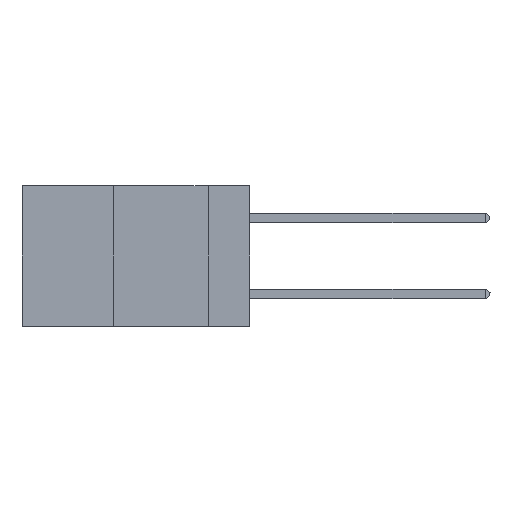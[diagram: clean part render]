
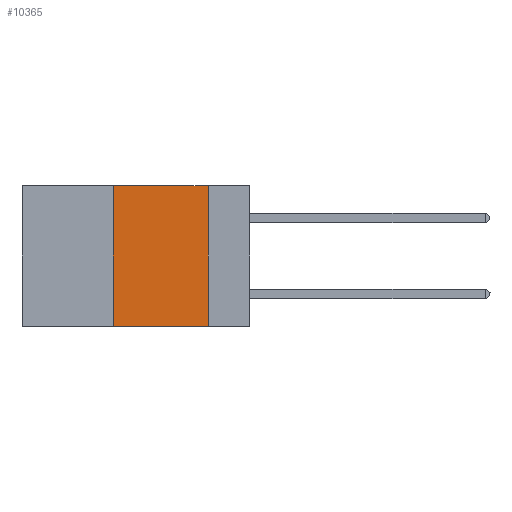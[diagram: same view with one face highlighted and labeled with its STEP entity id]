
A CAD part, left-side view. The second image highlights one B-rep face of the part: STEP entity #10365.
In plain terms, the highlighted planar face has unit normal (-1, 0, 0).
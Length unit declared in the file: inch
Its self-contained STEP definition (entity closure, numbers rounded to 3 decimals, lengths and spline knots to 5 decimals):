
#859 = ORIENTED_EDGE ( 'NONE', *, *, #12280, .F. ) ;
#2120 = CARTESIAN_POINT ( 'NONE',  ( 0., 0.36, 0. ) ) ;
#2125 = DIRECTION ( 'NONE',  ( 0., -1., 0. ) ) ;
#3086 = EDGE_CURVE ( 'NONE', #7713, #8307, #15124, .T. ) ;
#3375 = CARTESIAN_POINT ( 'NONE',  ( 0., 0.36, -0.37 ) ) ;
#3835 = ORIENTED_EDGE ( 'NONE', *, *, #3086, .F. ) ;
#4022 = LINE ( 'NONE', #10146, #11117 ) ;
#5123 = VERTEX_POINT ( 'NONE', #9319 ) ;
#5282 = EDGE_CURVE ( 'NONE', #7713, #5123, #4022, .T. ) ;
#5832 = VECTOR ( 'NONE', #16534, 39.37008 ) ;
#6125 = DIRECTION ( 'NONE',  ( 0., 0., -1. ) ) ;
#6964 = ORIENTED_EDGE ( 'NONE', *, *, #5282, .T. ) ;
#7713 = VERTEX_POINT ( 'NONE', #3375 ) ;
#7771 = EDGE_LOOP ( 'NONE', ( #859, #21436, #3835, #6964 ) ) ;
#8307 = VERTEX_POINT ( 'NONE', #10862 ) ;
#9319 = CARTESIAN_POINT ( 'NONE',  ( 0., 0.11, -0.37 ) ) ;
#9753 = EDGE_CURVE ( 'NONE', #8307, #19658, #16176, .T. ) ;
#9832 = CARTESIAN_POINT ( 'NONE',  ( 0., 0.6, 0. ) ) ;
#9899 = PLANE ( 'NONE',  #11299 ) ;
#10146 = CARTESIAN_POINT ( 'NONE',  ( 0., 0.6, -0.37 ) ) ;
#10365 = ADVANCED_FACE ( 'NONE', ( #22603 ), #9899, .F. ) ;
#10437 = LINE ( 'NONE', #18385, #11290 ) ;
#10862 = CARTESIAN_POINT ( 'NONE',  ( 0., 0.36, 0. ) ) ;
#11117 = VECTOR ( 'NONE', #18410, 39.37008 ) ;
#11290 = VECTOR ( 'NONE', #20188, 39.37008 ) ;
#11299 = AXIS2_PLACEMENT_3D ( 'NONE', #9832, #11740, #6125 ) ;
#11740 = DIRECTION ( 'NONE',  ( 1., 0., 0. ) ) ;
#12280 = EDGE_CURVE ( 'NONE', #19658, #5123, #10437, .T. ) ;
#12965 = CARTESIAN_POINT ( 'NONE',  ( 0., 0.6, 0. ) ) ;
#14128 = CARTESIAN_POINT ( 'NONE',  ( 0., 0.11, 0. ) ) ;
#15124 = LINE ( 'NONE', #2120, #5832 ) ;
#16176 = LINE ( 'NONE', #12965, #19278 ) ;
#16534 = DIRECTION ( 'NONE',  ( 0., 0., 1. ) ) ;
#18385 = CARTESIAN_POINT ( 'NONE',  ( 0., 0.11, 0. ) ) ;
#18410 = DIRECTION ( 'NONE',  ( 0., -1., 0. ) ) ;
#19278 = VECTOR ( 'NONE', #2125, 39.37008 ) ;
#19658 = VERTEX_POINT ( 'NONE', #14128 ) ;
#20188 = DIRECTION ( 'NONE',  ( 0., 0., -1. ) ) ;
#21436 = ORIENTED_EDGE ( 'NONE', *, *, #9753, .F. ) ;
#22603 = FACE_OUTER_BOUND ( 'NONE', #7771, .T. ) ;
